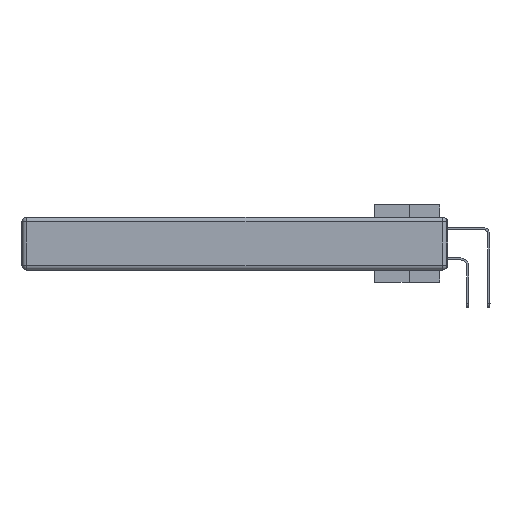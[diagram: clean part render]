
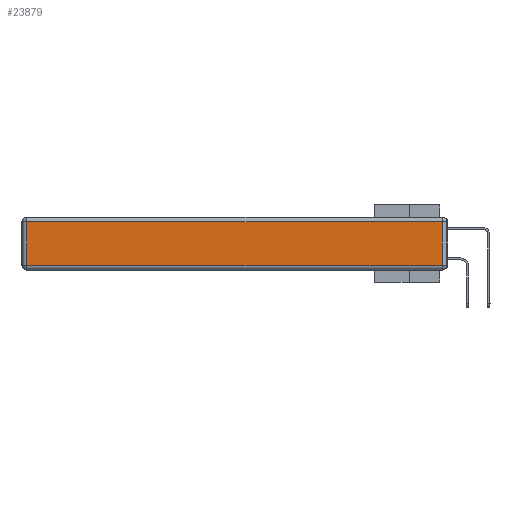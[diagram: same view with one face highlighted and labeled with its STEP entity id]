
A CAD part, left-side view. The second image highlights one B-rep face of the part: STEP entity #23879.
In plain terms, the highlighted planar face has unit normal (-1, 0, 0).
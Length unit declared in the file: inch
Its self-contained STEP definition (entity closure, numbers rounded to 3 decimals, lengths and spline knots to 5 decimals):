
#239 = CARTESIAN_POINT ( 'NONE',  ( 0., 0.03, -0.03 ) ) ;
#682 = CARTESIAN_POINT ( 'NONE',  ( 0., 2.72, -0.03 ) ) ;
#1872 = VECTOR ( 'NONE', #26746, 39.37008 ) ;
#3605 = DIRECTION ( 'NONE',  ( 0., 0., 1. ) ) ;
#6018 = DIRECTION ( 'NONE',  ( 0., -1., 0. ) ) ;
#7118 = AXIS2_PLACEMENT_3D ( 'NONE', #22805, #39198, #3605 ) ;
#9040 = ORIENTED_EDGE ( 'NONE', *, *, #11589, .T. ) ;
#11589 = EDGE_CURVE ( 'NONE', #37798, #22623, #14484, .T. ) ;
#12588 = ORIENTED_EDGE ( 'NONE', *, *, #34931, .T. ) ;
#12785 = CARTESIAN_POINT ( 'NONE',  ( 0., 2.72, -0.313 ) ) ;
#14063 = CARTESIAN_POINT ( 'NONE',  ( 0., 0.03, -0.313 ) ) ;
#14484 = LINE ( 'NONE', #40173, #26558 ) ;
#16692 = FACE_OUTER_BOUND ( 'NONE', #28797, .T. ) ;
#19424 = DIRECTION ( 'NONE',  ( 0., 0., 1. ) ) ;
#19582 = EDGE_CURVE ( 'NONE', #41454, #37798, #19833, .T. ) ;
#19833 = LINE ( 'NONE', #32250, #24554 ) ;
#20489 = VERTEX_POINT ( 'NONE', #12785 ) ;
#21407 = VECTOR ( 'NONE', #6018, 39.37008 ) ;
#22623 = VERTEX_POINT ( 'NONE', #682 ) ;
#22805 = CARTESIAN_POINT ( 'NONE',  ( 0., 0., -0.343 ) ) ;
#23879 = ADVANCED_FACE ( 'NONE', ( #16692 ), #29736, .T. ) ;
#24554 = VECTOR ( 'NONE', #19424, 39.37008 ) ;
#25709 = DIRECTION ( 'NONE',  ( 0., 1., 0. ) ) ;
#26558 = VECTOR ( 'NONE', #25709, 39.37008 ) ;
#26746 = DIRECTION ( 'NONE',  ( 0., 0., -1. ) ) ;
#28797 = EDGE_LOOP ( 'NONE', ( #35742, #38530, #9040, #12588 ) ) ;
#29736 = PLANE ( 'NONE',  #7118 ) ;
#30117 = CARTESIAN_POINT ( 'NONE',  ( 0., 2.72, -0.343 ) ) ;
#32250 = CARTESIAN_POINT ( 'NONE',  ( 0., 0.03, -0.343 ) ) ;
#34931 = EDGE_CURVE ( 'NONE', #22623, #20489, #39368, .T. ) ;
#35265 = LINE ( 'NONE', #41375, #21407 ) ;
#35632 = EDGE_CURVE ( 'NONE', #20489, #41454, #35265, .T. ) ;
#35742 = ORIENTED_EDGE ( 'NONE', *, *, #35632, .T. ) ;
#37798 = VERTEX_POINT ( 'NONE', #239 ) ;
#38530 = ORIENTED_EDGE ( 'NONE', *, *, #19582, .T. ) ;
#39198 = DIRECTION ( 'NONE',  ( -1., 0., 0. ) ) ;
#39368 = LINE ( 'NONE', #30117, #1872 ) ;
#40173 = CARTESIAN_POINT ( 'NONE',  ( 0., 2.75, -0.03 ) ) ;
#41375 = CARTESIAN_POINT ( 'NONE',  ( 0., 0., -0.313 ) ) ;
#41454 = VERTEX_POINT ( 'NONE', #14063 ) ;
